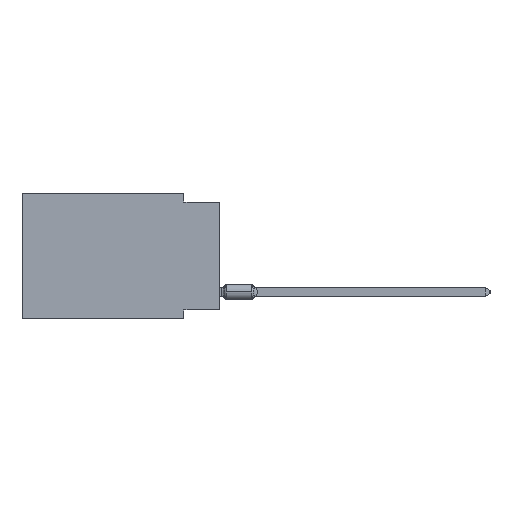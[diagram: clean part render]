
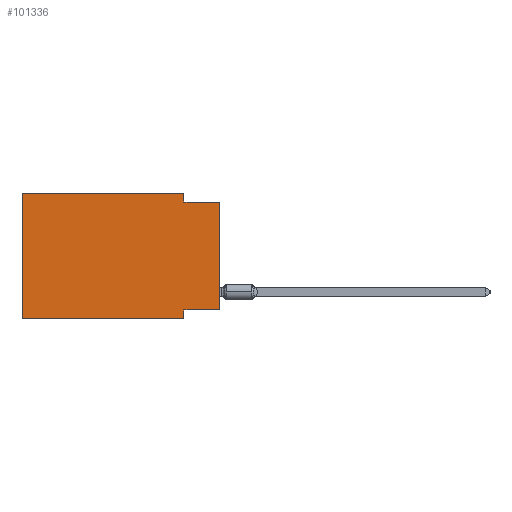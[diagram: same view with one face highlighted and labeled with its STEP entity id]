
A CAD part, left-side view. The second image highlights one B-rep face of the part: STEP entity #101336.
In plain terms, the highlighted planar face has unit normal (-1, 0, 0).
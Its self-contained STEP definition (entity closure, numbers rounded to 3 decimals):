
#288 = CARTESIAN_POINT ( 'NONE',  ( 0., 13.97, -8.89 ) ) ;
#1252 = EDGE_CURVE ( 'NONE', #57136, #54694, #90849, .T. ) ;
#2469 = ORIENTED_EDGE ( 'NONE', *, *, #83141, .T. ) ;
#6552 = DIRECTION ( 'NONE',  ( 0., 0., 1. ) ) ;
#7164 = ORIENTED_EDGE ( 'NONE', *, *, #50072, .T. ) ;
#8059 = VECTOR ( 'NONE', #25203, 1000. ) ;
#9054 = LINE ( 'NONE', #94855, #8059 ) ;
#13708 = FACE_OUTER_BOUND ( 'NONE', #77174, .T. ) ;
#17418 = CARTESIAN_POINT ( 'NONE',  ( 0., 2.54, -8.89 ) ) ;
#17558 = ORIENTED_EDGE ( 'NONE', *, *, #20990, .F. ) ;
#17964 = CARTESIAN_POINT ( 'NONE',  ( 0., 0., 0. ) ) ;
#20990 = EDGE_CURVE ( 'NONE', #87457, #57136, #69435, .T. ) ;
#25203 = DIRECTION ( 'NONE',  ( 0., 0., -1. ) ) ;
#26618 = CARTESIAN_POINT ( 'NONE',  ( 0., 0., -0.635 ) ) ;
#29734 = VECTOR ( 'NONE', #37003, 1000. ) ;
#31753 = CARTESIAN_POINT ( 'NONE',  ( 0., 2.54, -8.89 ) ) ;
#34322 = DIRECTION ( 'NONE',  ( 0., 1., 0. ) ) ;
#37003 = DIRECTION ( 'NONE',  ( 0., -1., 0. ) ) ;
#42343 = VECTOR ( 'NONE', #104894, 1000. ) ;
#42492 = CARTESIAN_POINT ( 'NONE',  ( 0., 2.54, 0. ) ) ;
#43274 = VERTEX_POINT ( 'NONE', #26618 ) ;
#44662 = ORIENTED_EDGE ( 'NONE', *, *, #75246, .F. ) ;
#45922 = CARTESIAN_POINT ( 'NONE',  ( 0., 13.97, 0. ) ) ;
#47698 = CARTESIAN_POINT ( 'NONE',  ( 0., 13.97, 0. ) ) ;
#49882 = DIRECTION ( 'NONE',  ( 0., 0., -1. ) ) ;
#50072 = EDGE_CURVE ( 'NONE', #87457, #43274, #78687, .T. ) ;
#50335 = AXIS2_PLACEMENT_3D ( 'NONE', #47698, #91705, #49882 ) ;
#50444 = LINE ( 'NONE', #288, #68171 ) ;
#54041 = VECTOR ( 'NONE', #34322, 1000. ) ;
#54694 = VERTEX_POINT ( 'NONE', #17418 ) ;
#54769 = VERTEX_POINT ( 'NONE', #42492 ) ;
#54951 = ORIENTED_EDGE ( 'NONE', *, *, #64839, .F. ) ;
#56163 = LINE ( 'NONE', #90159, #76922 ) ;
#57136 = VERTEX_POINT ( 'NONE', #72827 ) ;
#59358 = DIRECTION ( 'NONE',  ( 0., -1., 0. ) ) ;
#62942 = ORIENTED_EDGE ( 'NONE', *, *, #77246, .F. ) ;
#63244 = VECTOR ( 'NONE', #89751, 1000. ) ;
#64839 = EDGE_CURVE ( 'NONE', #86539, #75298, #56163, .T. ) ;
#68171 = VECTOR ( 'NONE', #59358, 1000. ) ;
#69435 = LINE ( 'NONE', #77250, #54041 ) ;
#72827 = CARTESIAN_POINT ( 'NONE',  ( 0., 2.54, -8.255 ) ) ;
#72916 = CARTESIAN_POINT ( 'NONE',  ( 0., 2.54, -0.635 ) ) ;
#75246 = EDGE_CURVE ( 'NONE', #75298, #54769, #95550, .T. ) ;
#75298 = VERTEX_POINT ( 'NONE', #45922 ) ;
#76922 = VECTOR ( 'NONE', #6552, 1000. ) ;
#77078 = CARTESIAN_POINT ( 'NONE',  ( 0., 0., -8.255 ) ) ;
#77174 = EDGE_LOOP ( 'NONE', ( #7164, #62942, #90380, #44662, #54951, #2469, #106550, #17558 ) ) ;
#77246 = EDGE_CURVE ( 'NONE', #99806, #43274, #103760, .T. ) ;
#77250 = CARTESIAN_POINT ( 'NONE',  ( 0., 0., -8.255 ) ) ;
#78266 = CARTESIAN_POINT ( 'NONE',  ( 0., 13.97, 0. ) ) ;
#78687 = LINE ( 'NONE', #17964, #42343 ) ;
#83141 = EDGE_CURVE ( 'NONE', #86539, #54694, #50444, .T. ) ;
#86539 = VERTEX_POINT ( 'NONE', #99804 ) ;
#87457 = VERTEX_POINT ( 'NONE', #77078 ) ;
#88693 = DIRECTION ( 'NONE',  ( 0., -1., 0. ) ) ;
#89751 = DIRECTION ( 'NONE',  ( 0., 0., -1. ) ) ;
#90159 = CARTESIAN_POINT ( 'NONE',  ( 0., 13.97, 0. ) ) ;
#90380 = ORIENTED_EDGE ( 'NONE', *, *, #92363, .F. ) ;
#90849 = LINE ( 'NONE', #31753, #63244 ) ;
#91705 = DIRECTION ( 'NONE',  ( 1., 0., 0. ) ) ;
#92363 = EDGE_CURVE ( 'NONE', #54769, #99806, #9054, .T. ) ;
#94855 = CARTESIAN_POINT ( 'NONE',  ( 0., 2.54, 0. ) ) ;
#95550 = LINE ( 'NONE', #78266, #29734 ) ;
#99804 = CARTESIAN_POINT ( 'NONE',  ( 0., 13.97, -8.89 ) ) ;
#99806 = VERTEX_POINT ( 'NONE', #72916 ) ;
#101336 = ADVANCED_FACE ( 'NONE', ( #13708 ), #108960, .F. ) ;
#101366 = VECTOR ( 'NONE', #88693, 1000. ) ;
#103760 = LINE ( 'NONE', #104311, #101366 ) ;
#104311 = CARTESIAN_POINT ( 'NONE',  ( 0., 0., -0.635 ) ) ;
#104894 = DIRECTION ( 'NONE',  ( 0., 0., 1. ) ) ;
#106550 = ORIENTED_EDGE ( 'NONE', *, *, #1252, .F. ) ;
#108960 = PLANE ( 'NONE',  #50335 ) ;
